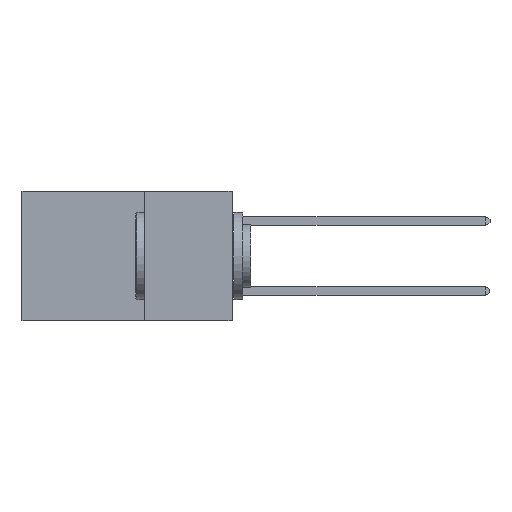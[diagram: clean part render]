
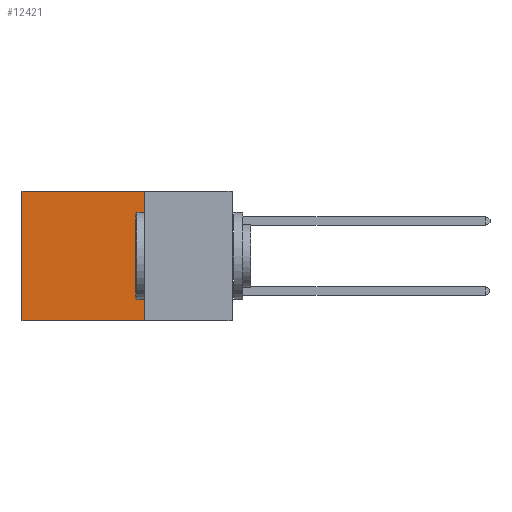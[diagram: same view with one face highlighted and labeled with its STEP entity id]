
A CAD part, left-side view. The second image highlights one B-rep face of the part: STEP entity #12421.
In plain terms, the highlighted planar face has unit normal (-1, 0, 0).
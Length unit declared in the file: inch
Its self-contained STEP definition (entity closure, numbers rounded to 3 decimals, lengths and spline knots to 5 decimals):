
#526 = CARTESIAN_POINT ( 'NONE',  ( 0.2875, 0.25, 0. ) ) ;
#685 = EDGE_CURVE ( 'NONE', #7479, #9211, #11690, .T. ) ;
#727 = CARTESIAN_POINT ( 'NONE',  ( 0.2875, 0.6, 0. ) ) ;
#999 = ORIENTED_EDGE ( 'NONE', *, *, #685, .F. ) ;
#1186 = DIRECTION ( 'NONE',  ( 0., 0., -1. ) ) ;
#1860 = CARTESIAN_POINT ( 'NONE',  ( 0.2875, 0.6, -0.37 ) ) ;
#2178 = ORIENTED_EDGE ( 'NONE', *, *, #3606, .F. ) ;
#2303 = LINE ( 'NONE', #16072, #8451 ) ;
#2781 = PLANE ( 'NONE',  #11968 ) ;
#2826 = LINE ( 'NONE', #12244, #15604 ) ;
#3604 = VECTOR ( 'NONE', #4852, 39.37008 ) ;
#3606 = EDGE_CURVE ( 'NONE', #9211, #14508, #9757, .T. ) ;
#4666 = VECTOR ( 'NONE', #1186, 39.37008 ) ;
#4697 = ORIENTED_EDGE ( 'NONE', *, *, #4839, .T. ) ;
#4811 = CARTESIAN_POINT ( 'NONE',  ( 0.2875, 0.25, -0.37 ) ) ;
#4839 = EDGE_CURVE ( 'NONE', #7479, #15701, #2826, .T. ) ;
#4852 = DIRECTION ( 'NONE',  ( 0., 1., 0. ) ) ;
#5262 = DIRECTION ( 'NONE',  ( 0., 0., -1. ) ) ;
#7188 = EDGE_CURVE ( 'NONE', #15701, #14508, #2303, .T. ) ;
#7479 = VERTEX_POINT ( 'NONE', #526 ) ;
#8451 = VECTOR ( 'NONE', #8601, 39.37008 ) ;
#8601 = DIRECTION ( 'NONE',  ( 0., 0., -1. ) ) ;
#9211 = VERTEX_POINT ( 'NONE', #12742 ) ;
#9757 = LINE ( 'NONE', #4811, #3604 ) ;
#10731 = CARTESIAN_POINT ( 'NONE',  ( 0.2875, 0.25, 0. ) ) ;
#11455 = CARTESIAN_POINT ( 'NONE',  ( 0.2875, 0.25, 0. ) ) ;
#11690 = LINE ( 'NONE', #10731, #4666 ) ;
#11790 = EDGE_LOOP ( 'NONE', ( #13471, #2178, #999, #4697 ) ) ;
#11968 = AXIS2_PLACEMENT_3D ( 'NONE', #11455, #12731, #5262 ) ;
#12187 = DIRECTION ( 'NONE',  ( 0., 1., 0. ) ) ;
#12244 = CARTESIAN_POINT ( 'NONE',  ( 0.2875, 0.25, 0. ) ) ;
#12421 = ADVANCED_FACE ( 'NONE', ( #14593 ), #2781, .F. ) ;
#12731 = DIRECTION ( 'NONE',  ( 1., 0., 0. ) ) ;
#12742 = CARTESIAN_POINT ( 'NONE',  ( 0.2875, 0.25, -0.37 ) ) ;
#13471 = ORIENTED_EDGE ( 'NONE', *, *, #7188, .T. ) ;
#14508 = VERTEX_POINT ( 'NONE', #1860 ) ;
#14593 = FACE_OUTER_BOUND ( 'NONE', #11790, .T. ) ;
#15604 = VECTOR ( 'NONE', #12187, 39.37008 ) ;
#15701 = VERTEX_POINT ( 'NONE', #727 ) ;
#16072 = CARTESIAN_POINT ( 'NONE',  ( 0.2875, 0.6, 0. ) ) ;
